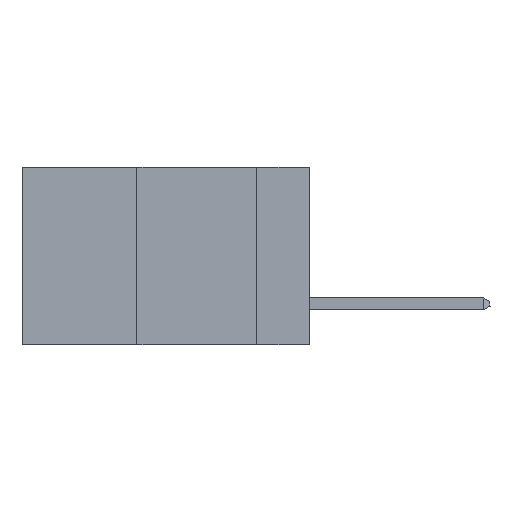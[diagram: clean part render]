
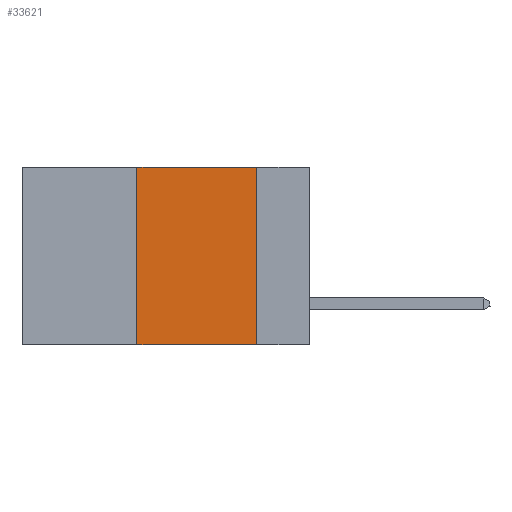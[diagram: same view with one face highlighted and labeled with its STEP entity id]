
A CAD part, left-side view. The second image highlights one B-rep face of the part: STEP entity #33621.
In plain terms, the highlighted planar face has unit normal (-1, 0, 0).
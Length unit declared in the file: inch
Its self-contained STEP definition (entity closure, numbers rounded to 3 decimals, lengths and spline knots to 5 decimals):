
#173 = VERTEX_POINT ( 'NONE', #1140 ) ;
#576 = CARTESIAN_POINT ( 'NONE',  ( 0., 0.36, 0. ) ) ;
#1140 = CARTESIAN_POINT ( 'NONE',  ( 0., 0.36, -0.37 ) ) ;
#3705 = LINE ( 'NONE', #10776, #28927 ) ;
#3765 = CARTESIAN_POINT ( 'NONE',  ( 0., 0.36, 0. ) ) ;
#4000 = VERTEX_POINT ( 'NONE', #3765 ) ;
#4042 = ORIENTED_EDGE ( 'NONE', *, *, #8396, .F. ) ;
#5814 = DIRECTION ( 'NONE',  ( 0., 0., -1. ) ) ;
#6134 = EDGE_CURVE ( 'NONE', #4000, #25380, #13364, .T. ) ;
#6489 = CARTESIAN_POINT ( 'NONE',  ( 0., 0.11, -0.37 ) ) ;
#7404 = EDGE_CURVE ( 'NONE', #173, #41529, #18465, .T. ) ;
#7805 = ORIENTED_EDGE ( 'NONE', *, *, #26345, .F. ) ;
#7866 = DIRECTION ( 'NONE',  ( 0., 0., -1. ) ) ;
#8396 = EDGE_CURVE ( 'NONE', #25380, #41529, #3705, .T. ) ;
#8457 = ORIENTED_EDGE ( 'NONE', *, *, #6134, .F. ) ;
#9315 = DIRECTION ( 'NONE',  ( 1., 0., 0. ) ) ;
#9393 = CARTESIAN_POINT ( 'NONE',  ( 0., 0.6, 0. ) ) ;
#10776 = CARTESIAN_POINT ( 'NONE',  ( 0., 0.11, 0. ) ) ;
#13364 = LINE ( 'NONE', #9393, #18045 ) ;
#15619 = FACE_OUTER_BOUND ( 'NONE', #17499, .T. ) ;
#17379 = ORIENTED_EDGE ( 'NONE', *, *, #7404, .T. ) ;
#17499 = EDGE_LOOP ( 'NONE', ( #4042, #8457, #7805, #17379 ) ) ;
#18045 = VECTOR ( 'NONE', #32905, 39.37008 ) ;
#18465 = LINE ( 'NONE', #36172, #31092 ) ;
#19427 = DIRECTION ( 'NONE',  ( 0., -1., 0. ) ) ;
#19899 = CARTESIAN_POINT ( 'NONE',  ( 0., 0.6, 0. ) ) ;
#24266 = VECTOR ( 'NONE', #24798, 39.37008 ) ;
#24798 = DIRECTION ( 'NONE',  ( 0., 0., 1. ) ) ;
#25380 = VERTEX_POINT ( 'NONE', #38396 ) ;
#26345 = EDGE_CURVE ( 'NONE', #173, #4000, #31606, .T. ) ;
#28927 = VECTOR ( 'NONE', #7866, 39.37008 ) ;
#31092 = VECTOR ( 'NONE', #19427, 39.37008 ) ;
#31606 = LINE ( 'NONE', #576, #24266 ) ;
#32905 = DIRECTION ( 'NONE',  ( 0., -1., 0. ) ) ;
#33621 = ADVANCED_FACE ( 'NONE', ( #15619 ), #43388, .F. ) ;
#33773 = AXIS2_PLACEMENT_3D ( 'NONE', #19899, #9315, #5814 ) ;
#36172 = CARTESIAN_POINT ( 'NONE',  ( 0., 0.6, -0.37 ) ) ;
#38396 = CARTESIAN_POINT ( 'NONE',  ( 0., 0.11, 0. ) ) ;
#41529 = VERTEX_POINT ( 'NONE', #6489 ) ;
#43388 = PLANE ( 'NONE',  #33773 ) ;
